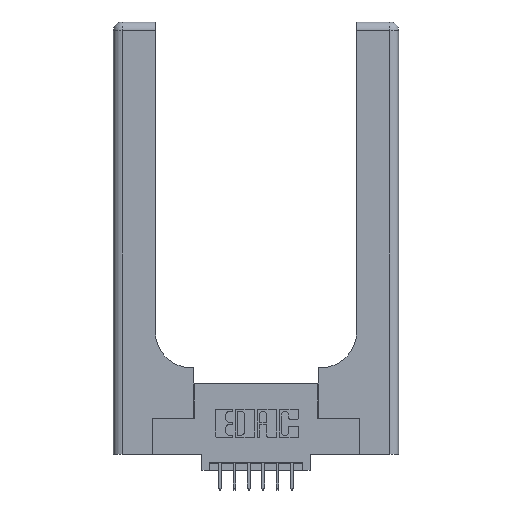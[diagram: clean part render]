
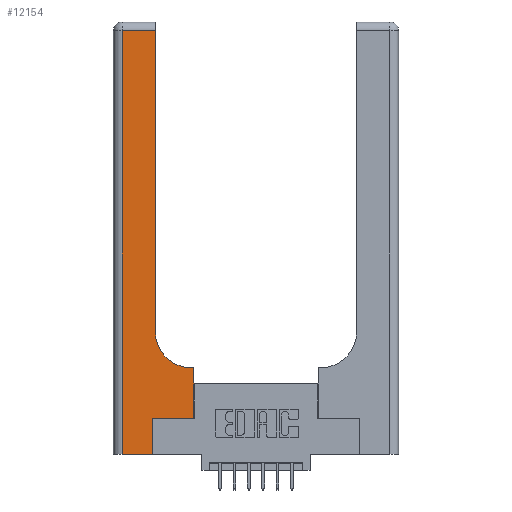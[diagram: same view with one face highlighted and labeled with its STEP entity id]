
A CAD part, top view. The second image highlights one B-rep face of the part: STEP entity #12154.
In plain terms, the highlighted planar face has unit normal (0, 0, 1).
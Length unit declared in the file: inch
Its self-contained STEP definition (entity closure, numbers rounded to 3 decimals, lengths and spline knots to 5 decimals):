
#2 = CARTESIAN_POINT ( 'NONE',  ( 0.269, 0., 0.37 ) ) ;
#818 = LINE ( 'NONE', #5407, #12144 ) ;
#860 = CARTESIAN_POINT ( 'NONE',  ( 0.06, 2.94, 0.37 ) ) ;
#937 = VERTEX_POINT ( 'NONE', #3515 ) ;
#952 = ORIENTED_EDGE ( 'NONE', *, *, #12169, .T. ) ;
#987 = CARTESIAN_POINT ( 'NONE',  ( 0., 3., 0.37 ) ) ;
#1268 = VERTEX_POINT ( 'NONE', #860 ) ;
#1476 = VERTEX_POINT ( 'NONE', #4917 ) ;
#2078 = CIRCLE ( 'NONE', #11029, 0.25 ) ;
#2401 = DIRECTION ( 'NONE',  ( 0., 0., -1. ) ) ;
#2974 = CARTESIAN_POINT ( 'NONE',  ( 0.2915, 0.6, 0.37 ) ) ;
#3066 = VERTEX_POINT ( 'NONE', #3397 ) ;
#3269 = LINE ( 'NONE', #7861, #10005 ) ;
#3278 = CARTESIAN_POINT ( 'NONE',  ( 0., 0., 0.37 ) ) ;
#3335 = CARTESIAN_POINT ( 'NONE',  ( 0., 2.94, 0.37 ) ) ;
#3397 = CARTESIAN_POINT ( 'NONE',  ( 0.5585, 0.6, 0.37 ) ) ;
#3488 = LINE ( 'NONE', #2, #10478 ) ;
#3515 = CARTESIAN_POINT ( 'NONE',  ( 0.06, 0., 0.37 ) ) ;
#3555 = VERTEX_POINT ( 'NONE', #14730 ) ;
#4212 = EDGE_CURVE ( 'NONE', #6140, #1476, #2078, .T. ) ;
#4309 = LINE ( 'NONE', #8212, #9804 ) ;
#4336 = LINE ( 'NONE', #2974, #9933 ) ;
#4608 = ORIENTED_EDGE ( 'NONE', *, *, #12481, .T. ) ;
#4916 = EDGE_CURVE ( 'NONE', #1268, #937, #4309, .T. ) ;
#4917 = CARTESIAN_POINT ( 'NONE',  ( 0.2915, 0.85, 0.37 ) ) ;
#5218 = DIRECTION ( 'NONE',  ( 1., 0., 0. ) ) ;
#5397 = ORIENTED_EDGE ( 'NONE', *, *, #8798, .T. ) ;
#5407 = CARTESIAN_POINT ( 'NONE',  ( 0.5585, 0.25, 0.37 ) ) ;
#5468 = DIRECTION ( 'NONE',  ( -1., 0., 0. ) ) ;
#5713 = ORIENTED_EDGE ( 'NONE', *, *, #12882, .T. ) ;
#5763 = CARTESIAN_POINT ( 'NONE',  ( 0.269, 0., 0.37 ) ) ;
#6140 = VERTEX_POINT ( 'NONE', #7801 ) ;
#6204 = CARTESIAN_POINT ( 'NONE',  ( 0.5585, 0.25, 0.37 ) ) ;
#6334 = LINE ( 'NONE', #10963, #11488 ) ;
#6740 = DIRECTION ( 'NONE',  ( 0., 1., 0. ) ) ;
#7041 = ORIENTED_EDGE ( 'NONE', *, *, #4212, .T. ) ;
#7801 = CARTESIAN_POINT ( 'NONE',  ( 0.5415, 0.6, 0.37 ) ) ;
#7861 = CARTESIAN_POINT ( 'NONE',  ( 0.2915, 3., 0.37 ) ) ;
#8212 = CARTESIAN_POINT ( 'NONE',  ( 0.06, 3., 0.37 ) ) ;
#8329 = VECTOR ( 'NONE', #14925, 39.37008 ) ;
#8382 = DIRECTION ( 'NONE',  ( 0., 1., 0. ) ) ;
#8540 = AXIS2_PLACEMENT_3D ( 'NONE', #987, #14845, #9074 ) ;
#8733 = EDGE_CURVE ( 'NONE', #3066, #6140, #4336, .T. ) ;
#8790 = ORIENTED_EDGE ( 'NONE', *, *, #13770, .T. ) ;
#8798 = EDGE_CURVE ( 'NONE', #937, #13322, #8933, .T. ) ;
#8933 = LINE ( 'NONE', #3278, #12589 ) ;
#8962 = VERTEX_POINT ( 'NONE', #6204 ) ;
#9074 = DIRECTION ( 'NONE',  ( -1., 0., 0. ) ) ;
#9076 = LINE ( 'NONE', #3335, #8329 ) ;
#9122 = ORIENTED_EDGE ( 'NONE', *, *, #8733, .T. ) ;
#9357 = DIRECTION ( 'NONE',  ( 1., 0., 0. ) ) ;
#9804 = VECTOR ( 'NONE', #11728, 39.37008 ) ;
#9864 = EDGE_CURVE ( 'NONE', #8962, #3066, #818, .T. ) ;
#9933 = VECTOR ( 'NONE', #5468, 39.37008 ) ;
#9944 = VERTEX_POINT ( 'NONE', #11847 ) ;
#10005 = VECTOR ( 'NONE', #6740, 39.37008 ) ;
#10031 = DIRECTION ( 'NONE',  ( 0., 1., 0. ) ) ;
#10320 = DIRECTION ( 'NONE',  ( 1., 0., 0. ) ) ;
#10478 = VECTOR ( 'NONE', #8382, 39.37008 ) ;
#10963 = CARTESIAN_POINT ( 'NONE',  ( 0.269, 0.25, 0.37 ) ) ;
#11029 = AXIS2_PLACEMENT_3D ( 'NONE', #12610, #2401, #9357 ) ;
#11099 = ORIENTED_EDGE ( 'NONE', *, *, #4916, .T. ) ;
#11355 = FACE_OUTER_BOUND ( 'NONE', #14582, .T. ) ;
#11488 = VECTOR ( 'NONE', #5218, 39.37008 ) ;
#11728 = DIRECTION ( 'NONE',  ( 0., -1., 0. ) ) ;
#11847 = CARTESIAN_POINT ( 'NONE',  ( 0.2915, 2.94, 0.37 ) ) ;
#12144 = VECTOR ( 'NONE', #10031, 39.37008 ) ;
#12154 = ADVANCED_FACE ( 'NONE', ( #11355 ), #13779, .F. ) ;
#12169 = EDGE_CURVE ( 'NONE', #13322, #3555, #3488, .T. ) ;
#12481 = EDGE_CURVE ( 'NONE', #1476, #9944, #3269, .T. ) ;
#12589 = VECTOR ( 'NONE', #10320, 39.37008 ) ;
#12610 = CARTESIAN_POINT ( 'NONE',  ( 0.5415, 0.85, 0.37 ) ) ;
#12882 = EDGE_CURVE ( 'NONE', #3555, #8962, #6334, .T. ) ;
#13322 = VERTEX_POINT ( 'NONE', #5763 ) ;
#13770 = EDGE_CURVE ( 'NONE', #9944, #1268, #9076, .T. ) ;
#13779 = PLANE ( 'NONE',  #8540 ) ;
#14232 = ORIENTED_EDGE ( 'NONE', *, *, #9864, .T. ) ;
#14582 = EDGE_LOOP ( 'NONE', ( #4608, #8790, #11099, #5397, #952, #5713, #14232, #9122, #7041 ) ) ;
#14730 = CARTESIAN_POINT ( 'NONE',  ( 0.269, 0.25, 0.37 ) ) ;
#14845 = DIRECTION ( 'NONE',  ( 0., 0., -1. ) ) ;
#14925 = DIRECTION ( 'NONE',  ( -1., 0., 0. ) ) ;
